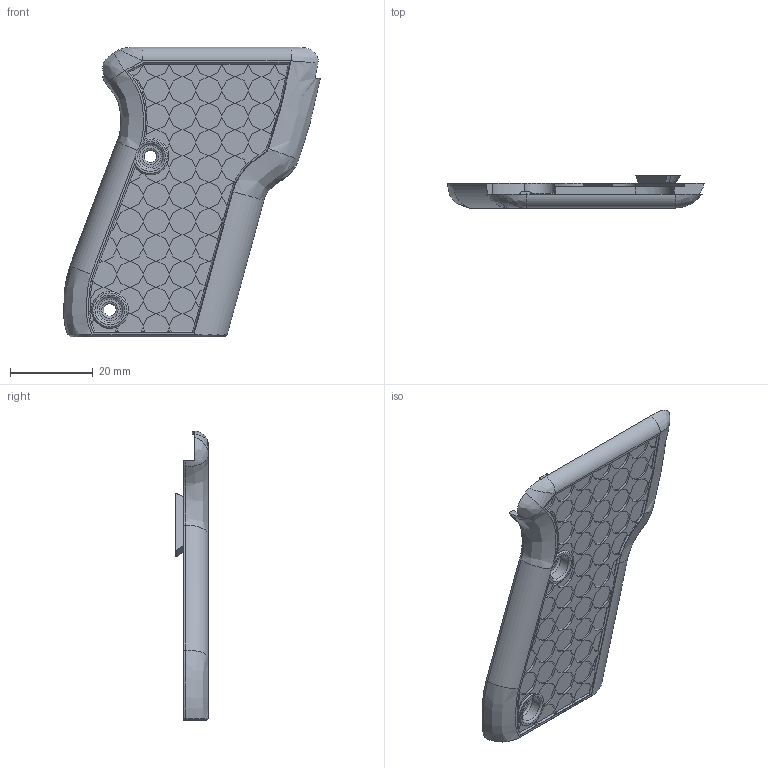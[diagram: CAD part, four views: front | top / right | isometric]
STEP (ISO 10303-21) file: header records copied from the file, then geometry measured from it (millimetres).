
FILE_DESCRIPTION(/* description */ (''),/* implementation_level */ '2;1');
FILE_NAME(/* name */ '21a-Grip-R-Final.step',/* time_stamp */ '2021-11-09T19:44:37-08:00',/* author */ (''),/* organization */ (''),/* preprocessor_version */ 'ST-DEVELOPER v18.1',/* originating_system */ 'Autodesk Translation Framework v10.10.0.1391',/* authorisation */ '');
FILE_SCHEMA (('AUTOMOTIVE_DESIGN { 1 0 10303 214 3 1 1 }'));
Length unit declared in the file: millimetre
Products named in the file (1): Grip-R-Final
Bounding box: 61.96 x 7.9 x 69.91 mm (x, y, z)
Volume: 12980.8 mm3; surface area: 8216.1 mm2
Topology: 1 solids, 1 shells, 569 faces, 1526 edges, 990 vertices
Faces by surface type: plane 486, bspline 51, cylinder 22, torus 8, cone 2
Full cylindrical faces by diameter (mm): 3 x2, 6.2 x2, 8.2 x1
Entity records: 20751 total; most frequent: CARTESIAN_POINT 6852, ORIENTED_EDGE 3050, DIRECTION 2513, EDGE_CURVE 1525, LINE 1315, VECTOR 1315, VERTEX_POINT 990, EDGE_LOOP 605
